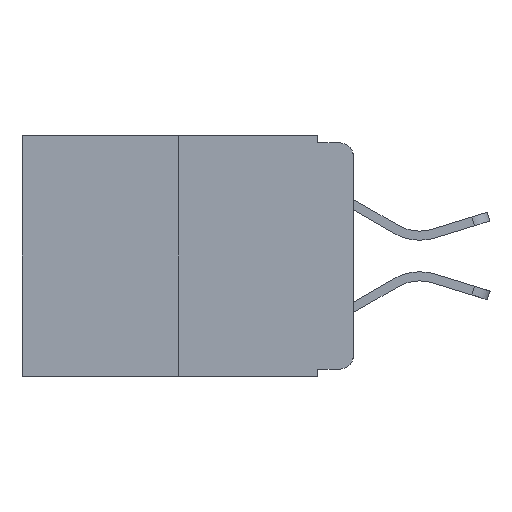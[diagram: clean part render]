
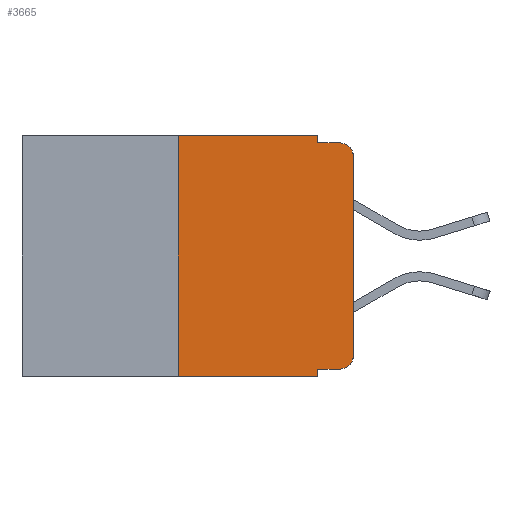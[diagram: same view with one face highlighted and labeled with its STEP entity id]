
A CAD part, left-side view. The second image highlights one B-rep face of the part: STEP entity #3665.
In plain terms, the highlighted planar face has unit normal (-1, 0, 0).
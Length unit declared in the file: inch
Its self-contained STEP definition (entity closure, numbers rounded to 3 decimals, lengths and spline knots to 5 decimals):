
#66 = CARTESIAN_POINT ( 'NONE',  ( 0., 0.051, 0. ) ) ;
#100 = EDGE_CURVE ( 'NONE', #8797, #3657, #1313, .T. ) ;
#186 = DIRECTION ( 'NONE',  ( 0., -1., 0. ) ) ;
#472 = DIRECTION ( 'NONE',  ( -1., 0., 0. ) ) ;
#581 = LINE ( 'NONE', #11968, #4768 ) ;
#868 = ORIENTED_EDGE ( 'NONE', *, *, #14058, .F. ) ;
#973 = DIRECTION ( 'NONE',  ( 0., 0., -1. ) ) ;
#1313 = LINE ( 'NONE', #3878, #3619 ) ;
#1326 = CARTESIAN_POINT ( 'NONE',  ( 0., 0.051, -0.01 ) ) ;
#1376 = DIRECTION ( 'NONE',  ( 0., 0., -1. ) ) ;
#1394 = DIRECTION ( 'NONE',  ( 0., 0., -1. ) ) ;
#1631 = VERTEX_POINT ( 'NONE', #1326 ) ;
#1946 = DIRECTION ( 'NONE',  ( 0., -1., 0. ) ) ;
#2516 = DIRECTION ( 'NONE',  ( 0., -1., 0. ) ) ;
#2559 = VERTEX_POINT ( 'NONE', #7449 ) ;
#3240 = DIRECTION ( 'NONE',  ( 0., 0., -1. ) ) ;
#3334 = ORIENTED_EDGE ( 'NONE', *, *, #9241, .T. ) ;
#3619 = VECTOR ( 'NONE', #4955, 39.37008 ) ;
#3657 = VERTEX_POINT ( 'NONE', #66 ) ;
#3665 = ADVANCED_FACE ( 'NONE', ( #7921 ), #12410, .F. ) ;
#3731 = LINE ( 'NONE', #8663, #6052 ) ;
#3742 = DIRECTION ( 'NONE',  ( 1., 0., 0. ) ) ;
#3829 = VERTEX_POINT ( 'NONE', #10512 ) ;
#3878 = CARTESIAN_POINT ( 'NONE',  ( 0., 0.473, 0. ) ) ;
#4216 = AXIS2_PLACEMENT_3D ( 'NONE', #12548, #472, #6466 ) ;
#4484 = LINE ( 'NONE', #10730, #15752 ) ;
#4537 = DIRECTION ( 'NONE',  ( 0., 0., 1. ) ) ;
#4577 = AXIS2_PLACEMENT_3D ( 'NONE', #15016, #3742, #1394 ) ;
#4582 = ORIENTED_EDGE ( 'NONE', *, *, #100, .F. ) ;
#4768 = VECTOR ( 'NONE', #4537, 39.37008 ) ;
#4955 = DIRECTION ( 'NONE',  ( 0., -1., 0. ) ) ;
#5073 = EDGE_CURVE ( 'NONE', #5273, #8797, #15476, .T. ) ;
#5273 = VERTEX_POINT ( 'NONE', #15925 ) ;
#6052 = VECTOR ( 'NONE', #186, 39.37008 ) ;
#6466 = DIRECTION ( 'NONE',  ( 0., 0., -1. ) ) ;
#6871 = CARTESIAN_POINT ( 'NONE',  ( 0., 0., -0.313 ) ) ;
#7004 = CARTESIAN_POINT ( 'NONE',  ( 0., 0.051, 0. ) ) ;
#7040 = VECTOR ( 'NONE', #2516, 39.37008 ) ;
#7449 = CARTESIAN_POINT ( 'NONE',  ( 0., 0.051, -0.333 ) ) ;
#7636 = EDGE_CURVE ( 'NONE', #5273, #3829, #3731, .T. ) ;
#7921 = FACE_OUTER_BOUND ( 'NONE', #9403, .T. ) ;
#8029 = EDGE_CURVE ( 'NONE', #3657, #1631, #4484, .T. ) ;
#8584 = DIRECTION ( 'NONE',  ( -1., 0., 0. ) ) ;
#8663 = CARTESIAN_POINT ( 'NONE',  ( 0., 0.473, -0.343 ) ) ;
#8751 = CARTESIAN_POINT ( 'NONE',  ( 0., 0.02, -0.313 ) ) ;
#8797 = VERTEX_POINT ( 'NONE', #15980 ) ;
#9182 = DIRECTION ( 'NONE',  ( 0., 0., 1. ) ) ;
#9241 = EDGE_CURVE ( 'NONE', #2559, #11760, #12412, .T. ) ;
#9242 = ORIENTED_EDGE ( 'NONE', *, *, #10880, .T. ) ;
#9367 = CIRCLE ( 'NONE', #11184, 0.02 ) ;
#9369 = VERTEX_POINT ( 'NONE', #14583 ) ;
#9403 = EDGE_LOOP ( 'NONE', ( #9242, #14511, #15142, #11052, #4582, #10284, #13360, #868, #3334, #14572 ) ) ;
#9934 = CARTESIAN_POINT ( 'NONE',  ( 0., 0.051, -0.01 ) ) ;
#9960 = VERTEX_POINT ( 'NONE', #6871 ) ;
#9999 = CARTESIAN_POINT ( 'NONE',  ( 0., 0.25, 0. ) ) ;
#10284 = ORIENTED_EDGE ( 'NONE', *, *, #5073, .F. ) ;
#10512 = CARTESIAN_POINT ( 'NONE',  ( 0., 0.051, -0.343 ) ) ;
#10730 = CARTESIAN_POINT ( 'NONE',  ( 0., 0.051, 0. ) ) ;
#10880 = EDGE_CURVE ( 'NONE', #9960, #9369, #581, .T. ) ;
#11052 = ORIENTED_EDGE ( 'NONE', *, *, #8029, .F. ) ;
#11184 = AXIS2_PLACEMENT_3D ( 'NONE', #8751, #8584, #1376 ) ;
#11760 = VERTEX_POINT ( 'NONE', #12028 ) ;
#11888 = CARTESIAN_POINT ( 'NONE',  ( 0., 0.051, -0.333 ) ) ;
#11915 = CIRCLE ( 'NONE', #4216, 0.02 ) ;
#11954 = EDGE_CURVE ( 'NONE', #9369, #13695, #11915, .T. ) ;
#11968 = CARTESIAN_POINT ( 'NONE',  ( 0., 0., 0. ) ) ;
#12028 = CARTESIAN_POINT ( 'NONE',  ( 0., 0.02, -0.333 ) ) ;
#12082 = LINE ( 'NONE', #9934, #7040 ) ;
#12410 = PLANE ( 'NONE',  #4577 ) ;
#12412 = LINE ( 'NONE', #11888, #15339 ) ;
#12548 = CARTESIAN_POINT ( 'NONE',  ( 0., 0.02, -0.03 ) ) ;
#12562 = LINE ( 'NONE', #7004, #12936 ) ;
#12725 = CARTESIAN_POINT ( 'NONE',  ( 0., 0.02, -0.01 ) ) ;
#12936 = VECTOR ( 'NONE', #3240, 39.37008 ) ;
#13360 = ORIENTED_EDGE ( 'NONE', *, *, #7636, .T. ) ;
#13506 = EDGE_CURVE ( 'NONE', #1631, #13695, #12082, .T. ) ;
#13576 = EDGE_CURVE ( 'NONE', #11760, #9960, #9367, .T. ) ;
#13695 = VERTEX_POINT ( 'NONE', #12725 ) ;
#14058 = EDGE_CURVE ( 'NONE', #2559, #3829, #12562, .T. ) ;
#14511 = ORIENTED_EDGE ( 'NONE', *, *, #11954, .T. ) ;
#14572 = ORIENTED_EDGE ( 'NONE', *, *, #13576, .T. ) ;
#14583 = CARTESIAN_POINT ( 'NONE',  ( 0., 0., -0.03 ) ) ;
#14869 = VECTOR ( 'NONE', #9182, 39.37008 ) ;
#15016 = CARTESIAN_POINT ( 'NONE',  ( 0., 0.473, 0. ) ) ;
#15142 = ORIENTED_EDGE ( 'NONE', *, *, #13506, .F. ) ;
#15339 = VECTOR ( 'NONE', #1946, 39.37008 ) ;
#15476 = LINE ( 'NONE', #9999, #14869 ) ;
#15752 = VECTOR ( 'NONE', #973, 39.37008 ) ;
#15925 = CARTESIAN_POINT ( 'NONE',  ( 0., 0.25, -0.343 ) ) ;
#15980 = CARTESIAN_POINT ( 'NONE',  ( 0., 0.25, 0. ) ) ;
